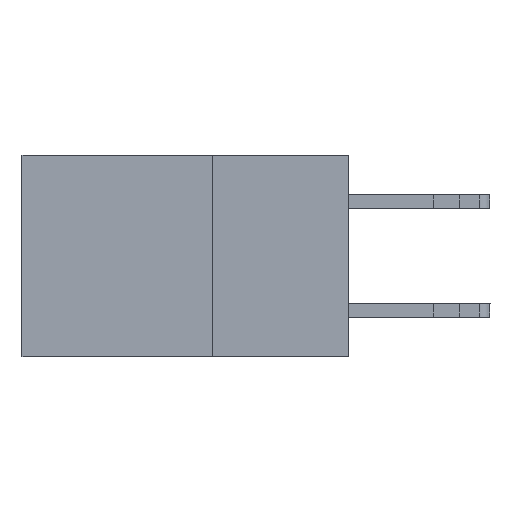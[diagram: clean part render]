
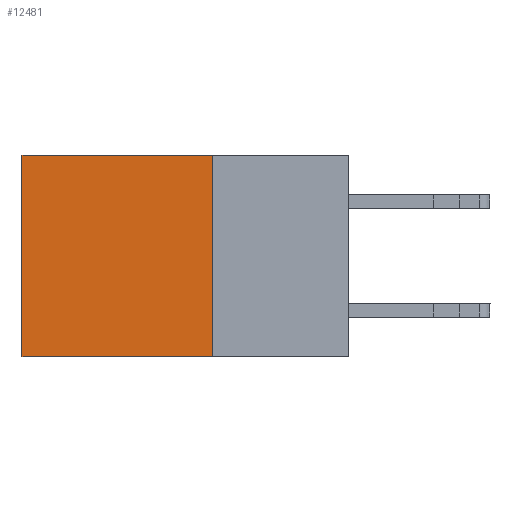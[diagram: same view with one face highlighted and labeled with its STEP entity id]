
A CAD part, left-side view. The second image highlights one B-rep face of the part: STEP entity #12481.
In plain terms, the highlighted planar face has unit normal (-1, 0, 0).
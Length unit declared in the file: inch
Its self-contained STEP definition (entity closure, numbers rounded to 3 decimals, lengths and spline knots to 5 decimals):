
#956 = EDGE_CURVE ( 'NONE', #10829, #2230, #4452, .T. ) ;
#1282 = ORIENTED_EDGE ( 'NONE', *, *, #12354, .T. ) ;
#1528 = VERTEX_POINT ( 'NONE', #9008 ) ;
#1671 = DIRECTION ( 'NONE',  ( 0., 0., -1. ) ) ;
#2230 = VERTEX_POINT ( 'NONE', #4262 ) ;
#3257 = ORIENTED_EDGE ( 'NONE', *, *, #4623, .F. ) ;
#3428 = LINE ( 'NONE', #7706, #9434 ) ;
#3444 = CARTESIAN_POINT ( 'NONE',  ( 0.2615, 0.25, -0.37 ) ) ;
#3470 = LINE ( 'NONE', #4438, #7389 ) ;
#3728 = FACE_OUTER_BOUND ( 'NONE', #7001, .T. ) ;
#4071 = VECTOR ( 'NONE', #1671, 39.37008 ) ;
#4262 = CARTESIAN_POINT ( 'NONE',  ( 0.2615, 0.6, -0.37 ) ) ;
#4420 = DIRECTION ( 'NONE',  ( 0., 1., 0. ) ) ;
#4438 = CARTESIAN_POINT ( 'NONE',  ( 0.2615, 0.25, -0.37 ) ) ;
#4452 = LINE ( 'NONE', #9524, #4071 ) ;
#4623 = EDGE_CURVE ( 'NONE', #12675, #2230, #3470, .T. ) ;
#4700 = DIRECTION ( 'NONE',  ( 1., 0., 0. ) ) ;
#5622 = CARTESIAN_POINT ( 'NONE',  ( 0.2615, 0.25, 0. ) ) ;
#5743 = CARTESIAN_POINT ( 'NONE',  ( 0.2615, 0.6, 0. ) ) ;
#7001 = EDGE_LOOP ( 'NONE', ( #10226, #3257, #13097, #1282 ) ) ;
#7389 = VECTOR ( 'NONE', #4420, 39.37008 ) ;
#7587 = DIRECTION ( 'NONE',  ( 0., 0., -1. ) ) ;
#7706 = CARTESIAN_POINT ( 'NONE',  ( 0.2615, 0.25, -0.37 ) ) ;
#8381 = LINE ( 'NONE', #5622, #13779 ) ;
#8694 = EDGE_CURVE ( 'NONE', #1528, #12675, #3428, .T. ) ;
#9008 = CARTESIAN_POINT ( 'NONE',  ( 0.2615, 0.25, 0. ) ) ;
#9434 = VECTOR ( 'NONE', #7587, 39.37008 ) ;
#9524 = CARTESIAN_POINT ( 'NONE',  ( 0.2615, 0.6, -0.37 ) ) ;
#10226 = ORIENTED_EDGE ( 'NONE', *, *, #956, .T. ) ;
#10829 = VERTEX_POINT ( 'NONE', #5743 ) ;
#12354 = EDGE_CURVE ( 'NONE', #1528, #10829, #8381, .T. ) ;
#12481 = ADVANCED_FACE ( 'NONE', ( #3728 ), #14956, .F. ) ;
#12675 = VERTEX_POINT ( 'NONE', #13122 ) ;
#12883 = DIRECTION ( 'NONE',  ( 0., 0., -1. ) ) ;
#13097 = ORIENTED_EDGE ( 'NONE', *, *, #8694, .F. ) ;
#13122 = CARTESIAN_POINT ( 'NONE',  ( 0.2615, 0.25, -0.37 ) ) ;
#13779 = VECTOR ( 'NONE', #14794, 39.37008 ) ;
#14794 = DIRECTION ( 'NONE',  ( 0., 1., 0. ) ) ;
#14956 = PLANE ( 'NONE',  #15099 ) ;
#15099 = AXIS2_PLACEMENT_3D ( 'NONE', #3444, #4700, #12883 ) ;
